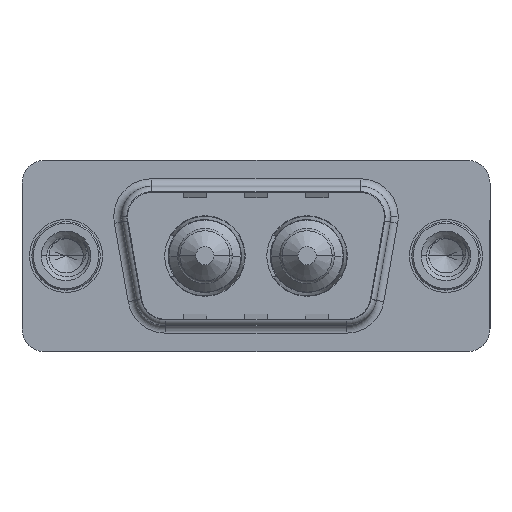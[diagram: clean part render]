
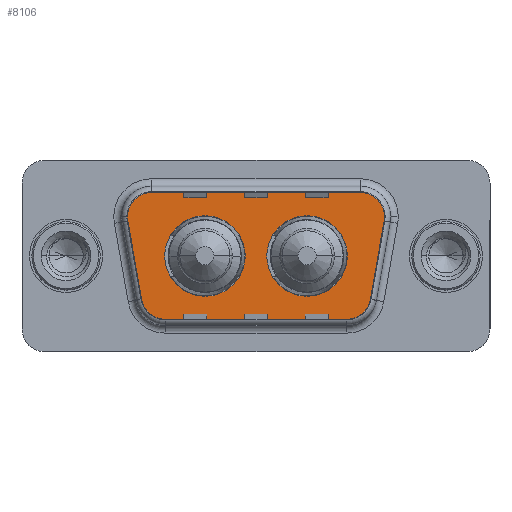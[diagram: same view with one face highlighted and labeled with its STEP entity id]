
A CAD part, top view. The second image highlights one B-rep face of the part: STEP entity #8106.
In plain terms, the highlighted planar face has unit normal (0, 0, 1).
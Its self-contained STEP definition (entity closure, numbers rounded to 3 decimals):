
#117 = ORIENTED_EDGE ( 'NONE', *, *, #9173, .F. ) ;
#317 = DIRECTION ( 'NONE',  ( 0., 0., 1. ) ) ;
#359 = VERTEX_POINT ( 'NONE', #5309 ) ;
#363 = EDGE_CURVE ( 'NONE', #12052, #944, #10654, .T. ) ;
#606 = FACE_BOUND ( 'NONE', #12897, .T. ) ;
#834 = CARTESIAN_POINT ( 'NONE',  ( 6.459, -4.9, 0. ) ) ;
#944 = VERTEX_POINT ( 'NONE', #6812 ) ;
#952 = LINE ( 'NONE', #10055, #8836 ) ;
#1152 = VERTEX_POINT ( 'NONE', #7041 ) ;
#1153 = DIRECTION ( 'NONE',  ( 0., 0., 1. ) ) ;
#1169 = CARTESIAN_POINT ( 'NONE',  ( 9.14, 0., 0. ) ) ;
#1256 = EDGE_CURVE ( 'NONE', #13340, #3664, #11774, .T. ) ;
#1381 = CARTESIAN_POINT ( 'NONE',  ( 11.79, 0., 0. ) ) ;
#1567 = CIRCLE ( 'NONE', #3376, 2.65 ) ;
#1675 = AXIS2_PLACEMENT_3D ( 'NONE', #13189, #12136, #12513 ) ;
#1976 = CARTESIAN_POINT ( 'NONE',  ( 3.466, 2.553, 0. ) ) ;
#1985 = EDGE_CURVE ( 'NONE', #4442, #12052, #952, .T. ) ;
#2154 = CARTESIAN_POINT ( 'NONE',  ( 6.459, -4.9, 0. ) ) ;
#2201 = ORIENTED_EDGE ( 'NONE', *, *, #8440, .T. ) ;
#2277 = EDGE_CURVE ( 'NONE', #8410, #12940, #11436, .T. ) ;
#2432 = ORIENTED_EDGE ( 'NONE', *, *, #2277, .T. ) ;
#2522 = CIRCLE ( 'NONE', #12292, 2.65 ) ;
#2606 = VERTEX_POINT ( 'NONE', #1381 ) ;
#2653 = ORIENTED_EDGE ( 'NONE', *, *, #1985, .T. ) ;
#2765 = CARTESIAN_POINT ( 'NONE',  ( 15.86, 0., 0. ) ) ;
#2977 = DIRECTION ( 'NONE',  ( 0., 0., 1. ) ) ;
#3013 = DIRECTION ( 'NONE',  ( 0., 0., 1. ) ) ;
#3030 = AXIS2_PLACEMENT_3D ( 'NONE', #3460, #317, #7593 ) ;
#3316 = CARTESIAN_POINT ( 'NONE',  ( 18.541, -4.9, 0. ) ) ;
#3376 = AXIS2_PLACEMENT_3D ( 'NONE', #7346, #1153, #8308 ) ;
#3460 = CARTESIAN_POINT ( 'NONE',  ( 18.541, -2.9, 0. ) ) ;
#3542 = VECTOR ( 'NONE', #7522, 1000. ) ;
#3664 = VERTEX_POINT ( 'NONE', #3316 ) ;
#3771 = DIRECTION ( 'NONE',  ( 1., 0., 0. ) ) ;
#3789 = AXIS2_PLACEMENT_3D ( 'NONE', #5310, #12473, #6393 ) ;
#4242 = EDGE_CURVE ( 'NONE', #4382, #2606, #5425, .T. ) ;
#4382 = VERTEX_POINT ( 'NONE', #5229 ) ;
#4423 = CARTESIAN_POINT ( 'NONE',  ( 5.436, 4.9, 0. ) ) ;
#4442 = VERTEX_POINT ( 'NONE', #9756 ) ;
#4477 = DIRECTION ( 'NONE',  ( 0., 0., 1. ) ) ;
#4585 = EDGE_CURVE ( 'NONE', #1152, #359, #8271, .T. ) ;
#4666 = CIRCLE ( 'NONE', #8240, 2. ) ;
#4744 = AXIS2_PLACEMENT_3D ( 'NONE', #1169, #13239, #13224 ) ;
#4901 = AXIS2_PLACEMENT_3D ( 'NONE', #5474, #11083, #13412 ) ;
#4930 = CIRCLE ( 'NONE', #4901, 2. ) ;
#5163 = ORIENTED_EDGE ( 'NONE', *, *, #8306, .F. ) ;
#5229 = CARTESIAN_POINT ( 'NONE',  ( 6.49, 0., 0. ) ) ;
#5309 = CARTESIAN_POINT ( 'NONE',  ( 4.489, -3.247, 0. ) ) ;
#5310 = CARTESIAN_POINT ( 'NONE',  ( 6.459, -2.9, 0. ) ) ;
#5319 = ORIENTED_EDGE ( 'NONE', *, *, #11869, .T. ) ;
#5425 = CIRCLE ( 'NONE', #4744, 2.65 ) ;
#5474 = CARTESIAN_POINT ( 'NONE',  ( 5.436, 2.9, 0. ) ) ;
#5599 = VERTEX_POINT ( 'NONE', #8446 ) ;
#5919 = EDGE_CURVE ( 'NONE', #12940, #1152, #4930, .T. ) ;
#6393 = DIRECTION ( 'NONE',  ( -1., 0., 0. ) ) ;
#6608 = PLANE ( 'NONE',  #3030 ) ;
#6812 = CARTESIAN_POINT ( 'NONE',  ( 21.564, 2.9, 0. ) ) ;
#7041 = CARTESIAN_POINT ( 'NONE',  ( 3.466, 2.553, 0. ) ) ;
#7315 = EDGE_CURVE ( 'NONE', #359, #13340, #8365, .T. ) ;
#7346 = CARTESIAN_POINT ( 'NONE',  ( 9.14, 0., 0. ) ) ;
#7364 = CARTESIAN_POINT ( 'NONE',  ( 21.534, 2.553, 0. ) ) ;
#7522 = DIRECTION ( 'NONE',  ( -1., 0., 0. ) ) ;
#7593 = DIRECTION ( 'NONE',  ( 1., 0., 0. ) ) ;
#7600 = ORIENTED_EDGE ( 'NONE', *, *, #12183, .F. ) ;
#7876 = FACE_OUTER_BOUND ( 'NONE', #10901, .T. ) ;
#8106 = ADVANCED_FACE ( 'NONE', ( #13018, #606, #7876 ), #6608, .T. ) ;
#8240 = AXIS2_PLACEMENT_3D ( 'NONE', #9121, #3013, #10189 ) ;
#8259 = DIRECTION ( 'NONE',  ( 0.174, -0.985, 0. ) ) ;
#8271 = LINE ( 'NONE', #1976, #10731 ) ;
#8306 = EDGE_CURVE ( 'NONE', #5599, #10273, #11431, .T. ) ;
#8308 = DIRECTION ( 'NONE',  ( 1., 0., 0. ) ) ;
#8365 = CIRCLE ( 'NONE', #3789, 2. ) ;
#8410 = VERTEX_POINT ( 'NONE', #12156 ) ;
#8440 = EDGE_CURVE ( 'NONE', #3664, #4442, #4666, .T. ) ;
#8446 = CARTESIAN_POINT ( 'NONE',  ( 13.21, 0., 0. ) ) ;
#8836 = VECTOR ( 'NONE', #12564, 1000. ) ;
#9045 = ORIENTED_EDGE ( 'NONE', *, *, #5919, .T. ) ;
#9080 = CARTESIAN_POINT ( 'NONE',  ( 19.564, 2.9, 0. ) ) ;
#9090 = AXIS2_PLACEMENT_3D ( 'NONE', #9080, #2977, #10142 ) ;
#9121 = CARTESIAN_POINT ( 'NONE',  ( 18.541, -2.9, 0. ) ) ;
#9173 = EDGE_CURVE ( 'NONE', #2606, #4382, #1567, .T. ) ;
#9318 = ORIENTED_EDGE ( 'NONE', *, *, #4242, .F. ) ;
#9330 = VECTOR ( 'NONE', #11285, 1000. ) ;
#9501 = EDGE_LOOP ( 'NONE', ( #7600, #5163 ) ) ;
#9720 = ORIENTED_EDGE ( 'NONE', *, *, #1256, .T. ) ;
#9756 = CARTESIAN_POINT ( 'NONE',  ( 20.511, -3.247, 0. ) ) ;
#9915 = DIRECTION ( 'NONE',  ( 0., 0., 1. ) ) ;
#10047 = CARTESIAN_POINT ( 'NONE',  ( 18.51, 0., 0. ) ) ;
#10055 = CARTESIAN_POINT ( 'NONE',  ( 21.534, 2.553, 0. ) ) ;
#10142 = DIRECTION ( 'NONE',  ( -1., 0., 0. ) ) ;
#10189 = DIRECTION ( 'NONE',  ( 1., 0., 0. ) ) ;
#10273 = VERTEX_POINT ( 'NONE', #10047 ) ;
#10372 = ORIENTED_EDGE ( 'NONE', *, *, #4585, .T. ) ;
#10604 = AXIS2_PLACEMENT_3D ( 'NONE', #2765, #9915, #3771 ) ;
#10640 = CARTESIAN_POINT ( 'NONE',  ( 15.86, 0., 0. ) ) ;
#10654 = CIRCLE ( 'NONE', #1675, 2. ) ;
#10695 = CARTESIAN_POINT ( 'NONE',  ( 5.436, 4.9, 0. ) ) ;
#10731 = VECTOR ( 'NONE', #8259, 1000. ) ;
#10901 = EDGE_LOOP ( 'NONE', ( #2201, #2653, #11638, #5319, #2432, #9045, #10372, #12147, #9720 ) ) ;
#11083 = DIRECTION ( 'NONE',  ( 0., 0., 1. ) ) ;
#11285 = DIRECTION ( 'NONE',  ( 1., 0., 0. ) ) ;
#11431 = CIRCLE ( 'NONE', #10604, 2.65 ) ;
#11436 = LINE ( 'NONE', #10695, #3542 ) ;
#11523 = CIRCLE ( 'NONE', #9090, 2. ) ;
#11638 = ORIENTED_EDGE ( 'NONE', *, *, #363, .T. ) ;
#11682 = DIRECTION ( 'NONE',  ( 1., 0., 0. ) ) ;
#11774 = LINE ( 'NONE', #2154, #9330 ) ;
#11869 = EDGE_CURVE ( 'NONE', #944, #8410, #11523, .T. ) ;
#12052 = VERTEX_POINT ( 'NONE', #7364 ) ;
#12136 = DIRECTION ( 'NONE',  ( 0., 0., 1. ) ) ;
#12147 = ORIENTED_EDGE ( 'NONE', *, *, #7315, .T. ) ;
#12156 = CARTESIAN_POINT ( 'NONE',  ( 19.564, 4.9, 0. ) ) ;
#12183 = EDGE_CURVE ( 'NONE', #10273, #5599, #2522, .T. ) ;
#12292 = AXIS2_PLACEMENT_3D ( 'NONE', #10640, #4477, #11682 ) ;
#12473 = DIRECTION ( 'NONE',  ( 0., 0., 1. ) ) ;
#12513 = DIRECTION ( 'NONE',  ( -1., 0., 0. ) ) ;
#12564 = DIRECTION ( 'NONE',  ( 0.174, 0.985, 0. ) ) ;
#12897 = EDGE_LOOP ( 'NONE', ( #117, #9318 ) ) ;
#12940 = VERTEX_POINT ( 'NONE', #4423 ) ;
#13018 = FACE_BOUND ( 'NONE', #9501, .T. ) ;
#13189 = CARTESIAN_POINT ( 'NONE',  ( 19.564, 2.9, 0. ) ) ;
#13224 = DIRECTION ( 'NONE',  ( 1., 0., 0. ) ) ;
#13239 = DIRECTION ( 'NONE',  ( 0., 0., 1. ) ) ;
#13340 = VERTEX_POINT ( 'NONE', #834 ) ;
#13412 = DIRECTION ( 'NONE',  ( 1., 0., 0. ) ) ;
